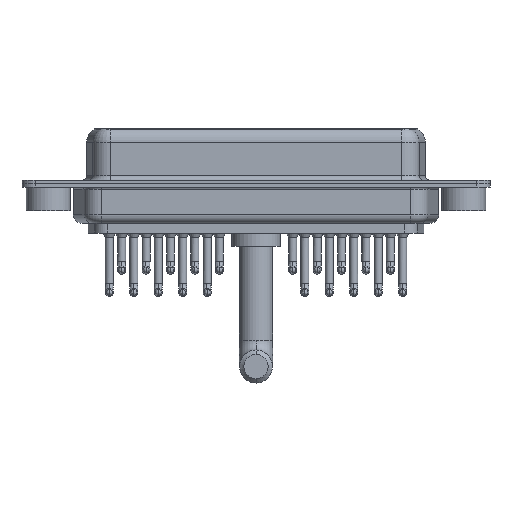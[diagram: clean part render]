
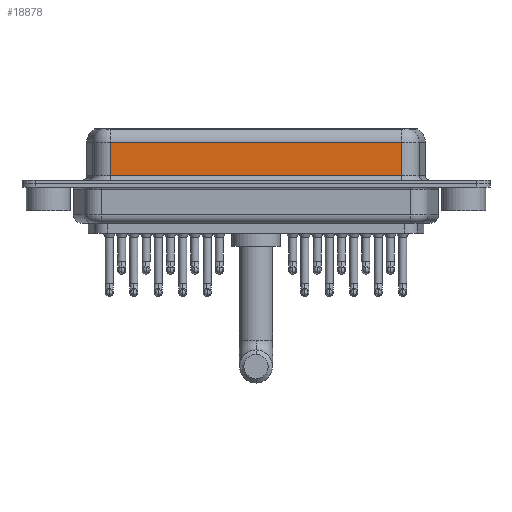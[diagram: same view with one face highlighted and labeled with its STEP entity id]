
A CAD part, front view. The second image highlights one B-rep face of the part: STEP entity #18878.
In plain terms, the highlighted planar face has unit normal (0, -1, 0).
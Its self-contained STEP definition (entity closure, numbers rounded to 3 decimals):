
#394 = CARTESIAN_POINT ( 'NONE',  ( 40.037, -3.95, 0.9 ) ) ;
#395 = EDGE_CURVE ( 'NONE', #2061, #5213, #10935, .T. ) ;
#487 = VERTEX_POINT ( 'NONE', #394 ) ;
#1481 = CARTESIAN_POINT ( 'NONE',  ( 40.037, -3.95, 6.4 ) ) ;
#1822 = VECTOR ( 'NONE', #10979, 1000. ) ;
#2061 = VERTEX_POINT ( 'NONE', #17333 ) ;
#3890 = EDGE_CURVE ( 'NONE', #5213, #487, #11105, .T. ) ;
#4525 = VECTOR ( 'NONE', #21236, 1000. ) ;
#4915 = PLANE ( 'NONE',  #12218 ) ;
#5213 = VERTEX_POINT ( 'NONE', #6521 ) ;
#6506 = DIRECTION ( 'NONE',  ( 0., 0., 1. ) ) ;
#6521 = CARTESIAN_POINT ( 'NONE',  ( 7.013, -3.95, 0.9 ) ) ;
#7283 = CARTESIAN_POINT ( 'NONE',  ( 40.037, -3.95, 4.65 ) ) ;
#8716 = DIRECTION ( 'NONE',  ( 0., 0., -1. ) ) ;
#10346 = CARTESIAN_POINT ( 'NONE',  ( 40.037, -3.95, 6.4 ) ) ;
#10868 = CARTESIAN_POINT ( 'NONE',  ( 40.037, -3.95, 0.9 ) ) ;
#10935 = LINE ( 'NONE', #17932, #4525 ) ;
#10979 = DIRECTION ( 'NONE',  ( 1., 0., 0. ) ) ;
#11105 = LINE ( 'NONE', #10868, #1822 ) ;
#11541 = ORIENTED_EDGE ( 'NONE', *, *, #12111, .T. ) ;
#11754 = EDGE_LOOP ( 'NONE', ( #17116, #11541, #19618, #19020 ) ) ;
#12056 = LINE ( 'NONE', #10346, #14083 ) ;
#12111 = EDGE_CURVE ( 'NONE', #22255, #2061, #14404, .T. ) ;
#12139 = FACE_OUTER_BOUND ( 'NONE', #11754, .T. ) ;
#12218 = AXIS2_PLACEMENT_3D ( 'NONE', #1481, #19123, #6506 ) ;
#14083 = VECTOR ( 'NONE', #8716, 1000. ) ;
#14404 = LINE ( 'NONE', #19649, #14674 ) ;
#14674 = VECTOR ( 'NONE', #17958, 1000. ) ;
#17116 = ORIENTED_EDGE ( 'NONE', *, *, #19868, .F. ) ;
#17333 = CARTESIAN_POINT ( 'NONE',  ( 7.013, -3.95, 4.65 ) ) ;
#17932 = CARTESIAN_POINT ( 'NONE',  ( 7.013, -3.95, 6.4 ) ) ;
#17958 = DIRECTION ( 'NONE',  ( -1., 0., 0. ) ) ;
#18878 = ADVANCED_FACE ( 'NONE', ( #12139 ), #4915, .F. ) ;
#19020 = ORIENTED_EDGE ( 'NONE', *, *, #3890, .T. ) ;
#19123 = DIRECTION ( 'NONE',  ( 0., 1., 0. ) ) ;
#19618 = ORIENTED_EDGE ( 'NONE', *, *, #395, .T. ) ;
#19649 = CARTESIAN_POINT ( 'NONE',  ( 40.037, -3.95, 4.65 ) ) ;
#19868 = EDGE_CURVE ( 'NONE', #22255, #487, #12056, .T. ) ;
#21236 = DIRECTION ( 'NONE',  ( 0., 0., -1. ) ) ;
#22255 = VERTEX_POINT ( 'NONE', #7283 ) ;
